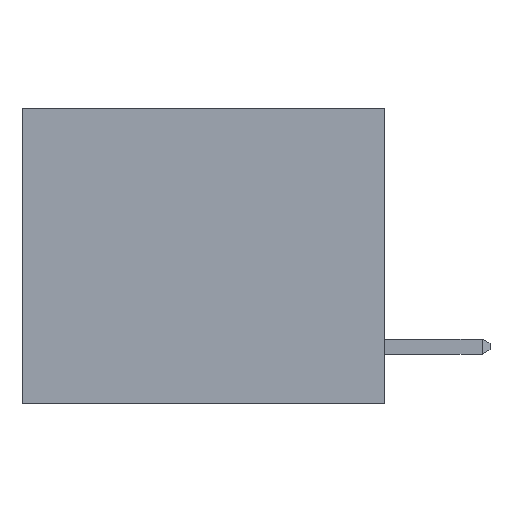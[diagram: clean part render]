
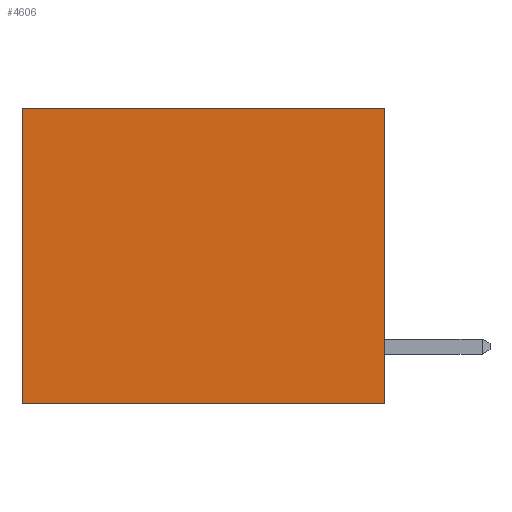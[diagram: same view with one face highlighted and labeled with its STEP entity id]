
A CAD part, left-side view. The second image highlights one B-rep face of the part: STEP entity #4606.
In plain terms, the highlighted planar face has unit normal (-1, 0, 0).
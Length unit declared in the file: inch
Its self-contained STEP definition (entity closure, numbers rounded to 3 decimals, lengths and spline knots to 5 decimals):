
#83 = EDGE_CURVE ( 'NONE', #1938, #289, #3181, .T. ) ;
#175 = LINE ( 'NONE', #5637, #4753 ) ;
#289 = VERTEX_POINT ( 'NONE', #3696 ) ;
#523 = CARTESIAN_POINT ( 'NONE',  ( 0.3165, 0., -0.49 ) ) ;
#838 = LINE ( 'NONE', #1245, #7275 ) ;
#1082 = AXIS2_PLACEMENT_3D ( 'NONE', #5049, #5620, #2129 ) ;
#1245 = CARTESIAN_POINT ( 'NONE',  ( 0.3165, 0., -0.49 ) ) ;
#1342 = EDGE_CURVE ( 'NONE', #4209, #289, #175, .T. ) ;
#1417 = EDGE_CURVE ( 'NONE', #4386, #4209, #5102, .T. ) ;
#1938 = VERTEX_POINT ( 'NONE', #523 ) ;
#2129 = DIRECTION ( 'NONE',  ( 0., 0., -1. ) ) ;
#2483 = ORIENTED_EDGE ( 'NONE', *, *, #1417, .T. ) ;
#3181 = LINE ( 'NONE', #3453, #4358 ) ;
#3453 = CARTESIAN_POINT ( 'NONE',  ( 0.3165, 0., -0.49 ) ) ;
#3696 = CARTESIAN_POINT ( 'NONE',  ( 0.3165, 0.6, -0.49 ) ) ;
#3831 = ORIENTED_EDGE ( 'NONE', *, *, #83, .F. ) ;
#4035 = DIRECTION ( 'NONE',  ( 0., 1., 0. ) ) ;
#4085 = EDGE_CURVE ( 'NONE', #4386, #1938, #838, .T. ) ;
#4164 = DIRECTION ( 'NONE',  ( 0., 0., -1. ) ) ;
#4209 = VERTEX_POINT ( 'NONE', #6266 ) ;
#4219 = CARTESIAN_POINT ( 'NONE',  ( 0.3165, 0., 0. ) ) ;
#4358 = VECTOR ( 'NONE', #4035, 39.37008 ) ;
#4386 = VERTEX_POINT ( 'NONE', #4219 ) ;
#4463 = DIRECTION ( 'NONE',  ( 0., 1., 0. ) ) ;
#4502 = ORIENTED_EDGE ( 'NONE', *, *, #4085, .F. ) ;
#4606 = ADVANCED_FACE ( 'NONE', ( #6149 ), #7382, .F. ) ;
#4753 = VECTOR ( 'NONE', #6241, 39.37008 ) ;
#5049 = CARTESIAN_POINT ( 'NONE',  ( 0.3165, 0., -0.49 ) ) ;
#5102 = LINE ( 'NONE', #6778, #5538 ) ;
#5538 = VECTOR ( 'NONE', #4463, 39.37008 ) ;
#5620 = DIRECTION ( 'NONE',  ( 1., 0., 0. ) ) ;
#5637 = CARTESIAN_POINT ( 'NONE',  ( 0.3165, 0.6, -0.49 ) ) ;
#6122 = EDGE_LOOP ( 'NONE', ( #6541, #3831, #4502, #2483 ) ) ;
#6149 = FACE_OUTER_BOUND ( 'NONE', #6122, .T. ) ;
#6241 = DIRECTION ( 'NONE',  ( 0., 0., -1. ) ) ;
#6266 = CARTESIAN_POINT ( 'NONE',  ( 0.3165, 0.6, 0. ) ) ;
#6541 = ORIENTED_EDGE ( 'NONE', *, *, #1342, .T. ) ;
#6778 = CARTESIAN_POINT ( 'NONE',  ( 0.3165, 0., 0. ) ) ;
#7275 = VECTOR ( 'NONE', #4164, 39.37008 ) ;
#7382 = PLANE ( 'NONE',  #1082 ) ;
